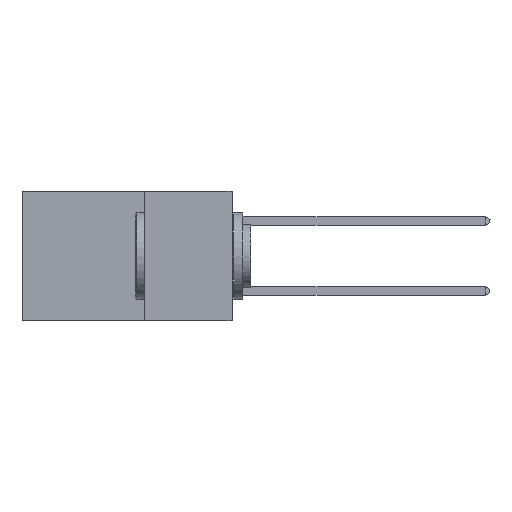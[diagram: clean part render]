
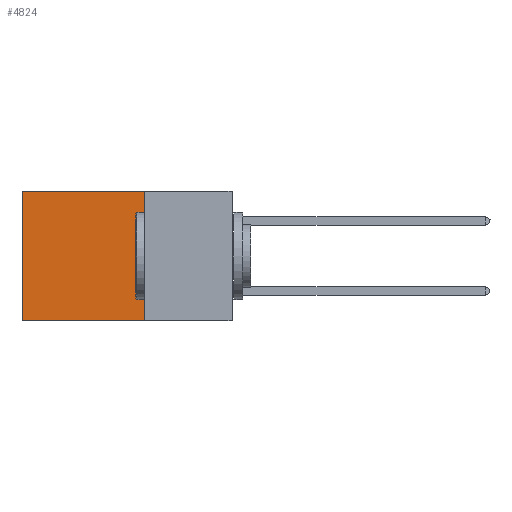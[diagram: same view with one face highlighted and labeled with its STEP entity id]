
A CAD part, left-side view. The second image highlights one B-rep face of the part: STEP entity #4824.
In plain terms, the highlighted planar face has unit normal (-1, 0, 0).
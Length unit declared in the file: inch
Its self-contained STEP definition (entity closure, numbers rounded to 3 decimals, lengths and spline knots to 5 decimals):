
#492 = ORIENTED_EDGE ( 'NONE', *, *, #12198, .T. ) ;
#2057 = VECTOR ( 'NONE', #16213, 39.37008 ) ;
#2653 = FACE_OUTER_BOUND ( 'NONE', #11371, .T. ) ;
#3170 = LINE ( 'NONE', #15460, #12662 ) ;
#4020 = ORIENTED_EDGE ( 'NONE', *, *, #5935, .T. ) ;
#4528 = CARTESIAN_POINT ( 'NONE',  ( 0.2875, 0.6, -0.37 ) ) ;
#4824 = ADVANCED_FACE ( 'NONE', ( #2653 ), #6899, .F. ) ;
#4910 = VERTEX_POINT ( 'NONE', #18629 ) ;
#5148 = CARTESIAN_POINT ( 'NONE',  ( 0.2875, 0.25, -0.37 ) ) ;
#5935 = EDGE_CURVE ( 'NONE', #4910, #11696, #11890, .T. ) ;
#6843 = DIRECTION ( 'NONE',  ( 0., 0., -1. ) ) ;
#6899 = PLANE ( 'NONE',  #15755 ) ;
#7405 = CARTESIAN_POINT ( 'NONE',  ( 0.2875, 0.25, -0.37 ) ) ;
#7940 = VERTEX_POINT ( 'NONE', #10936 ) ;
#9005 = LINE ( 'NONE', #7405, #11013 ) ;
#10621 = VERTEX_POINT ( 'NONE', #5148 ) ;
#10868 = LINE ( 'NONE', #11867, #2057 ) ;
#10936 = CARTESIAN_POINT ( 'NONE',  ( 0.2875, 0.25, 0. ) ) ;
#11003 = CARTESIAN_POINT ( 'NONE',  ( 0.2875, 0.25, 0. ) ) ;
#11013 = VECTOR ( 'NONE', #13168, 39.37008 ) ;
#11371 = EDGE_LOOP ( 'NONE', ( #4020, #13368, #11651, #492 ) ) ;
#11505 = DIRECTION ( 'NONE',  ( 0., 0., -1. ) ) ;
#11651 = ORIENTED_EDGE ( 'NONE', *, *, #12473, .F. ) ;
#11696 = VERTEX_POINT ( 'NONE', #4528 ) ;
#11867 = CARTESIAN_POINT ( 'NONE',  ( 0.2875, 0.25, 0. ) ) ;
#11890 = LINE ( 'NONE', #15433, #17960 ) ;
#12198 = EDGE_CURVE ( 'NONE', #7940, #4910, #10868, .T. ) ;
#12473 = EDGE_CURVE ( 'NONE', #7940, #10621, #3170, .T. ) ;
#12662 = VECTOR ( 'NONE', #11505, 39.37008 ) ;
#13168 = DIRECTION ( 'NONE',  ( 0., 1., 0. ) ) ;
#13368 = ORIENTED_EDGE ( 'NONE', *, *, #17680, .F. ) ;
#14046 = DIRECTION ( 'NONE',  ( 0., 0., -1. ) ) ;
#15291 = DIRECTION ( 'NONE',  ( 1., 0., 0. ) ) ;
#15433 = CARTESIAN_POINT ( 'NONE',  ( 0.2875, 0.6, 0. ) ) ;
#15460 = CARTESIAN_POINT ( 'NONE',  ( 0.2875, 0.25, 0. ) ) ;
#15755 = AXIS2_PLACEMENT_3D ( 'NONE', #11003, #15291, #14046 ) ;
#16213 = DIRECTION ( 'NONE',  ( 0., 1., 0. ) ) ;
#17680 = EDGE_CURVE ( 'NONE', #10621, #11696, #9005, .T. ) ;
#17960 = VECTOR ( 'NONE', #6843, 39.37008 ) ;
#18629 = CARTESIAN_POINT ( 'NONE',  ( 0.2875, 0.6, 0. ) ) ;
